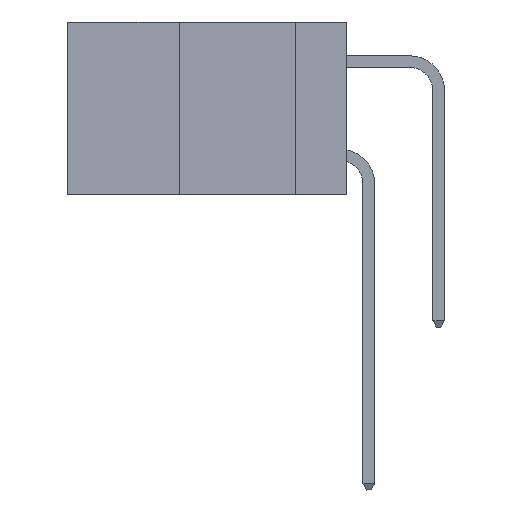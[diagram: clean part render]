
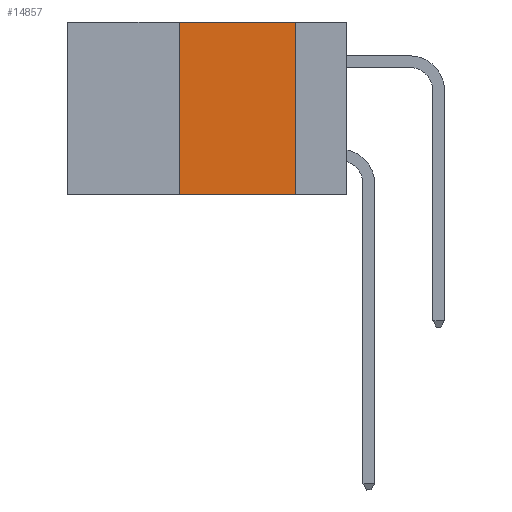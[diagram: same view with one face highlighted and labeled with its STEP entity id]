
A CAD part, left-side view. The second image highlights one B-rep face of the part: STEP entity #14857.
In plain terms, the highlighted planar face has unit normal (-1, 0, 0).
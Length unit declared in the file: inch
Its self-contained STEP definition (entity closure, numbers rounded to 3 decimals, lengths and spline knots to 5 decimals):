
#516 = LINE ( 'NONE', #3184, #15270 ) ;
#1526 = DIRECTION ( 'NONE',  ( 0., -1., 0. ) ) ;
#1651 = DIRECTION ( 'NONE',  ( 0., 0., 1. ) ) ;
#1751 = CARTESIAN_POINT ( 'NONE',  ( 0., 0.11, 0. ) ) ;
#2069 = EDGE_LOOP ( 'NONE', ( #7014, #16552, #3809, #8587 ) ) ;
#3184 = CARTESIAN_POINT ( 'NONE',  ( 0., 0.11, 0. ) ) ;
#3809 = ORIENTED_EDGE ( 'NONE', *, *, #8147, .F. ) ;
#4204 = EDGE_CURVE ( 'NONE', #8443, #6641, #16721, .T. ) ;
#4886 = VERTEX_POINT ( 'NONE', #1751 ) ;
#5506 = DIRECTION ( 'NONE',  ( 1., 0., 0. ) ) ;
#5679 = CARTESIAN_POINT ( 'NONE',  ( 0., 0.6, -0.37 ) ) ;
#6062 = EDGE_CURVE ( 'NONE', #16824, #4886, #11894, .T. ) ;
#6641 = VERTEX_POINT ( 'NONE', #11454 ) ;
#7014 = ORIENTED_EDGE ( 'NONE', *, *, #17364, .F. ) ;
#7145 = DIRECTION ( 'NONE',  ( 0., -1., 0. ) ) ;
#8147 = EDGE_CURVE ( 'NONE', #8443, #16824, #12891, .T. ) ;
#8236 = VECTOR ( 'NONE', #1526, 39.37008 ) ;
#8443 = VERTEX_POINT ( 'NONE', #9813 ) ;
#8587 = ORIENTED_EDGE ( 'NONE', *, *, #4204, .T. ) ;
#8829 = CARTESIAN_POINT ( 'NONE',  ( 0., 0.6, 0. ) ) ;
#9260 = VECTOR ( 'NONE', #1651, 39.37008 ) ;
#9813 = CARTESIAN_POINT ( 'NONE',  ( 0., 0.36, -0.37 ) ) ;
#11127 = PLANE ( 'NONE',  #14983 ) ;
#11454 = CARTESIAN_POINT ( 'NONE',  ( 0., 0.11, -0.37 ) ) ;
#11894 = LINE ( 'NONE', #8829, #8236 ) ;
#12891 = LINE ( 'NONE', #15807, #9260 ) ;
#13041 = VECTOR ( 'NONE', #7145, 39.37008 ) ;
#13652 = FACE_OUTER_BOUND ( 'NONE', #2069, .T. ) ;
#13882 = CARTESIAN_POINT ( 'NONE',  ( 0., 0.6, 0. ) ) ;
#14066 = CARTESIAN_POINT ( 'NONE',  ( 0., 0.36, 0. ) ) ;
#14857 = ADVANCED_FACE ( 'NONE', ( #13652 ), #11127, .F. ) ;
#14983 = AXIS2_PLACEMENT_3D ( 'NONE', #13882, #5506, #15276 ) ;
#15270 = VECTOR ( 'NONE', #15909, 39.37008 ) ;
#15276 = DIRECTION ( 'NONE',  ( 0., 0., -1. ) ) ;
#15807 = CARTESIAN_POINT ( 'NONE',  ( 0., 0.36, 0. ) ) ;
#15909 = DIRECTION ( 'NONE',  ( 0., 0., -1. ) ) ;
#16552 = ORIENTED_EDGE ( 'NONE', *, *, #6062, .F. ) ;
#16721 = LINE ( 'NONE', #5679, #13041 ) ;
#16824 = VERTEX_POINT ( 'NONE', #14066 ) ;
#17364 = EDGE_CURVE ( 'NONE', #4886, #6641, #516, .T. ) ;
